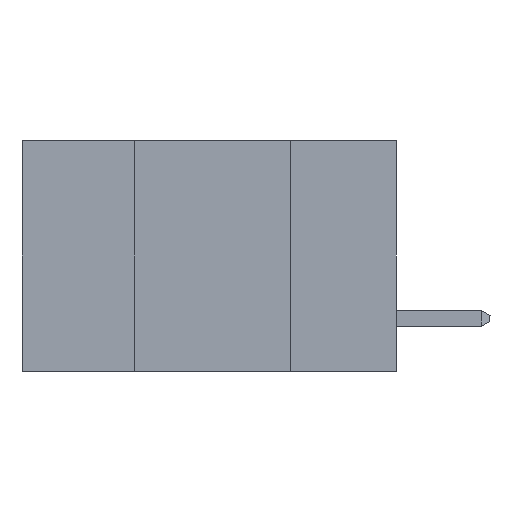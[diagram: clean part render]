
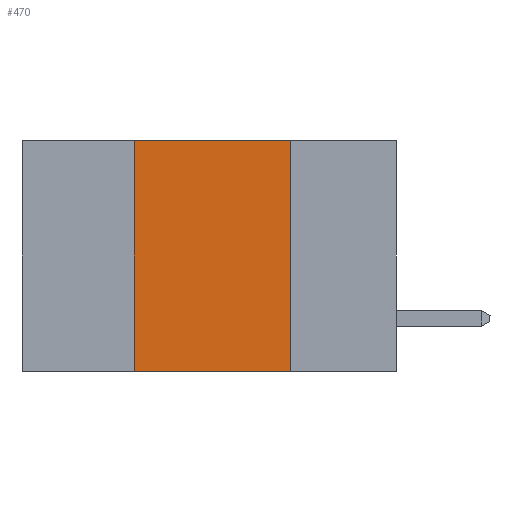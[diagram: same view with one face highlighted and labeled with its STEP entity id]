
A CAD part, left-side view. The second image highlights one B-rep face of the part: STEP entity #470.
In plain terms, the highlighted planar face has unit normal (-1, 0, 0).
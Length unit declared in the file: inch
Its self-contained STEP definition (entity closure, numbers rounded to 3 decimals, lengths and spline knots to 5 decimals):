
#343 = VERTEX_POINT ( 'NONE', #10638 ) ;
#470 = ADVANCED_FACE ( 'NONE', ( #1899 ), #10040, .F. ) ;
#1364 = ORIENTED_EDGE ( 'NONE', *, *, #8081, .T. ) ;
#1899 = FACE_OUTER_BOUND ( 'NONE', #7894, .T. ) ;
#2345 = LINE ( 'NONE', #5215, #8294 ) ;
#2543 = LINE ( 'NONE', #5686, #10821 ) ;
#2823 = VERTEX_POINT ( 'NONE', #6090 ) ;
#2842 = EDGE_CURVE ( 'NONE', #8802, #10106, #2543, .T. ) ;
#3636 = DIRECTION ( 'NONE',  ( 0., -1., 0. ) ) ;
#3952 = ORIENTED_EDGE ( 'NONE', *, *, #2842, .F. ) ;
#4116 = LINE ( 'NONE', #5842, #5987 ) ;
#4521 = DIRECTION ( 'NONE',  ( 0., 0., -1. ) ) ;
#5215 = CARTESIAN_POINT ( 'NONE',  ( 0., 0.6, -0.37 ) ) ;
#5329 = DIRECTION ( 'NONE',  ( 0., 0., -1. ) ) ;
#5587 = DIRECTION ( 'NONE',  ( 0., -1., 0. ) ) ;
#5686 = CARTESIAN_POINT ( 'NONE',  ( 0., 0.6, 0. ) ) ;
#5842 = CARTESIAN_POINT ( 'NONE',  ( 0., 0.42, -0.37 ) ) ;
#5987 = VECTOR ( 'NONE', #8315, 39.37008 ) ;
#6054 = AXIS2_PLACEMENT_3D ( 'NONE', #6373, #6428, #5329 ) ;
#6070 = ORIENTED_EDGE ( 'NONE', *, *, #9759, .F. ) ;
#6090 = CARTESIAN_POINT ( 'NONE',  ( 0., 0.17, -0.37 ) ) ;
#6373 = CARTESIAN_POINT ( 'NONE',  ( 0., 0.6, 0. ) ) ;
#6428 = DIRECTION ( 'NONE',  ( 1., 0., 0. ) ) ;
#6724 = LINE ( 'NONE', #8589, #10736 ) ;
#7274 = CARTESIAN_POINT ( 'NONE',  ( 0., 0.17, 0. ) ) ;
#7877 = EDGE_CURVE ( 'NONE', #343, #8802, #4116, .T. ) ;
#7894 = EDGE_LOOP ( 'NONE', ( #6070, #3952, #8017, #1364 ) ) ;
#8017 = ORIENTED_EDGE ( 'NONE', *, *, #7877, .F. ) ;
#8081 = EDGE_CURVE ( 'NONE', #343, #2823, #2345, .T. ) ;
#8294 = VECTOR ( 'NONE', #3636, 39.37008 ) ;
#8315 = DIRECTION ( 'NONE',  ( 0., 0., 1. ) ) ;
#8589 = CARTESIAN_POINT ( 'NONE',  ( 0., 0.17, -0.37 ) ) ;
#8802 = VERTEX_POINT ( 'NONE', #10165 ) ;
#9759 = EDGE_CURVE ( 'NONE', #10106, #2823, #6724, .T. ) ;
#10040 = PLANE ( 'NONE',  #6054 ) ;
#10106 = VERTEX_POINT ( 'NONE', #7274 ) ;
#10165 = CARTESIAN_POINT ( 'NONE',  ( 0., 0.42, 0. ) ) ;
#10638 = CARTESIAN_POINT ( 'NONE',  ( 0., 0.42, -0.37 ) ) ;
#10736 = VECTOR ( 'NONE', #4521, 39.37008 ) ;
#10821 = VECTOR ( 'NONE', #5587, 39.37008 ) ;
